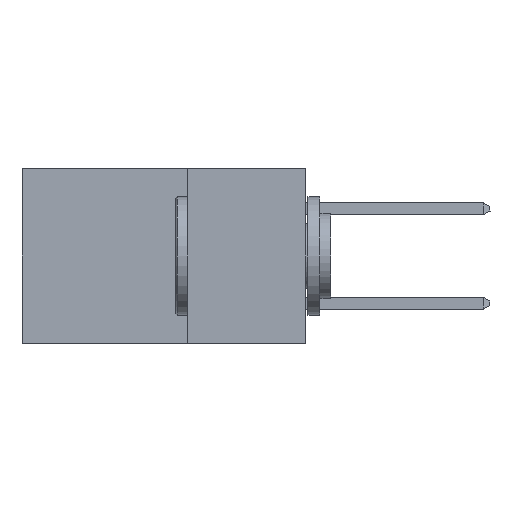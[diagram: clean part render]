
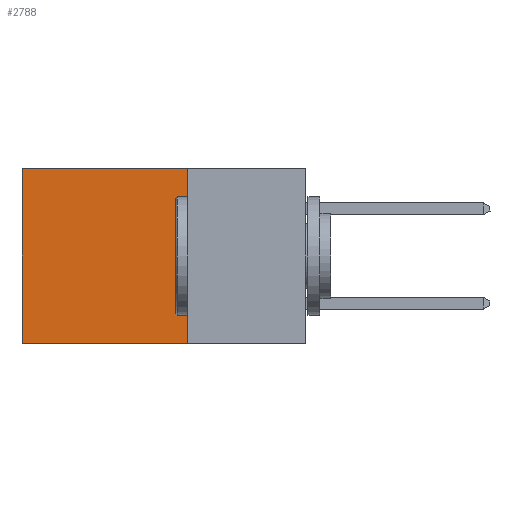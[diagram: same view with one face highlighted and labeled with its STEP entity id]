
A CAD part, left-side view. The second image highlights one B-rep face of the part: STEP entity #2788.
In plain terms, the highlighted planar face has unit normal (-1, 0, 0).
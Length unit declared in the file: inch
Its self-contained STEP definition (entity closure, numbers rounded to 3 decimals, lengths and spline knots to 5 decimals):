
#463 = DIRECTION ( 'NONE',  ( 0., 0., -1. ) ) ;
#1075 = CARTESIAN_POINT ( 'NONE',  ( 0.298, 0.25, -0.37 ) ) ;
#1139 = PLANE ( 'NONE',  #1965 ) ;
#1217 = LINE ( 'NONE', #8409, #5040 ) ;
#1332 = VERTEX_POINT ( 'NONE', #5334 ) ;
#1662 = FACE_OUTER_BOUND ( 'NONE', #3739, .T. ) ;
#1675 = EDGE_CURVE ( 'NONE', #6814, #6541, #9035, .T. ) ;
#1965 = AXIS2_PLACEMENT_3D ( 'NONE', #7236, #3658, #6328 ) ;
#1994 = VECTOR ( 'NONE', #4669, 39.37008 ) ;
#2104 = CARTESIAN_POINT ( 'NONE',  ( 0.298, 0.6, 0. ) ) ;
#2788 = ADVANCED_FACE ( 'NONE', ( #1662 ), #1139, .F. ) ;
#3554 = ORIENTED_EDGE ( 'NONE', *, *, #7201, .T. ) ;
#3658 = DIRECTION ( 'NONE',  ( 1., 0., 0. ) ) ;
#3739 = EDGE_LOOP ( 'NONE', ( #3554, #6145, #7864, #4469 ) ) ;
#4213 = LINE ( 'NONE', #7681, #6395 ) ;
#4469 = ORIENTED_EDGE ( 'NONE', *, *, #4683, .T. ) ;
#4507 = CARTESIAN_POINT ( 'NONE',  ( 0.298, 0.6, 0. ) ) ;
#4669 = DIRECTION ( 'NONE',  ( 0., 0., -1. ) ) ;
#4683 = EDGE_CURVE ( 'NONE', #6814, #10616, #4213, .T. ) ;
#5040 = VECTOR ( 'NONE', #9280, 39.37008 ) ;
#5091 = CARTESIAN_POINT ( 'NONE',  ( 0.298, 0.25, 0. ) ) ;
#5334 = CARTESIAN_POINT ( 'NONE',  ( 0.298, 0.6, -0.37 ) ) ;
#6145 = ORIENTED_EDGE ( 'NONE', *, *, #10810, .F. ) ;
#6328 = DIRECTION ( 'NONE',  ( 0., 0., -1. ) ) ;
#6395 = VECTOR ( 'NONE', #9426, 39.37008 ) ;
#6541 = VERTEX_POINT ( 'NONE', #1075 ) ;
#6742 = VECTOR ( 'NONE', #463, 39.37008 ) ;
#6814 = VERTEX_POINT ( 'NONE', #5091 ) ;
#7201 = EDGE_CURVE ( 'NONE', #10616, #1332, #11261, .T. ) ;
#7236 = CARTESIAN_POINT ( 'NONE',  ( 0.298, 0.25, 0. ) ) ;
#7681 = CARTESIAN_POINT ( 'NONE',  ( 0.298, 0.25, 0. ) ) ;
#7864 = ORIENTED_EDGE ( 'NONE', *, *, #1675, .F. ) ;
#8209 = CARTESIAN_POINT ( 'NONE',  ( 0.298, 0.25, 0. ) ) ;
#8409 = CARTESIAN_POINT ( 'NONE',  ( 0.298, 0.25, -0.37 ) ) ;
#9035 = LINE ( 'NONE', #8209, #6742 ) ;
#9280 = DIRECTION ( 'NONE',  ( 0., 1., 0. ) ) ;
#9426 = DIRECTION ( 'NONE',  ( 0., 1., 0. ) ) ;
#10616 = VERTEX_POINT ( 'NONE', #4507 ) ;
#10810 = EDGE_CURVE ( 'NONE', #6541, #1332, #1217, .T. ) ;
#11261 = LINE ( 'NONE', #2104, #1994 ) ;
